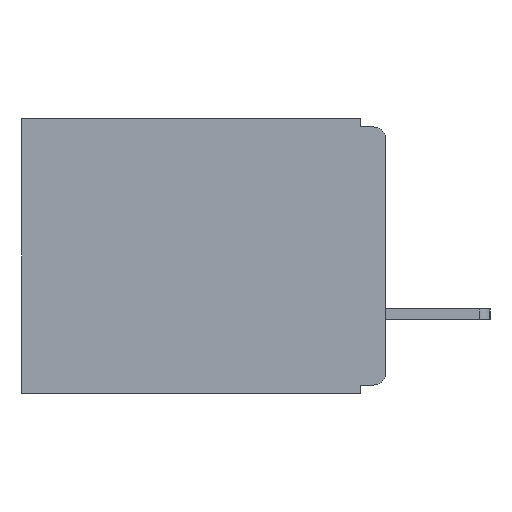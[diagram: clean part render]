
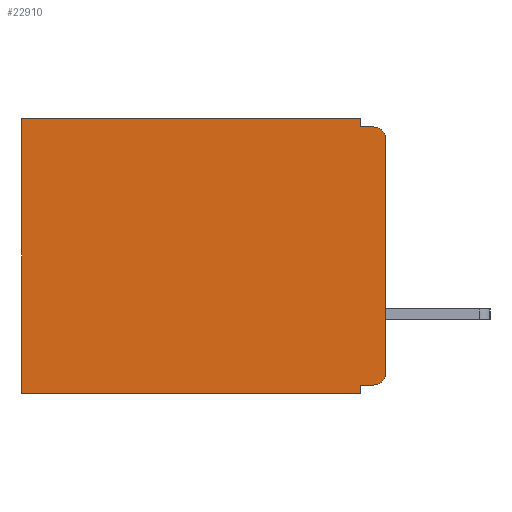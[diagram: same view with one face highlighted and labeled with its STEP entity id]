
A CAD part, left-side view. The second image highlights one B-rep face of the part: STEP entity #22910.
In plain terms, the highlighted planar face has unit normal (-1, 0, 0).
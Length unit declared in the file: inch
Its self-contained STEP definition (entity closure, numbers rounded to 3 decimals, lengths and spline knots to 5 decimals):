
#33 = EDGE_CURVE ( 'NONE', #7114, #3083, #21932, .T. ) ;
#176 = ORIENTED_EDGE ( 'NONE', *, *, #8968, .T. ) ;
#306 = LINE ( 'NONE', #16758, #4225 ) ;
#610 = CARTESIAN_POINT ( 'NONE',  ( 0.3, 0., -0.33 ) ) ;
#956 = EDGE_LOOP ( 'NONE', ( #25468, #28493, #5058, #9358, #176, #7870, #13820, #5344, #19461, #2371 ) ) ;
#1788 = VERTEX_POINT ( 'NONE', #25112 ) ;
#1789 = LINE ( 'NONE', #610, #13122 ) ;
#2048 = CARTESIAN_POINT ( 'NONE',  ( 0.3, 0.437, 0. ) ) ;
#2189 = CARTESIAN_POINT ( 'NONE',  ( 0.3, 0., -0.33 ) ) ;
#2371 = ORIENTED_EDGE ( 'NONE', *, *, #14044, .T. ) ;
#3065 = CIRCLE ( 'NONE', #7094, 0.015 ) ;
#3083 = VERTEX_POINT ( 'NONE', #17396 ) ;
#3307 = VECTOR ( 'NONE', #19195, 39.37008 ) ;
#3341 = CARTESIAN_POINT ( 'NONE',  ( 0.3, 0., -0.32 ) ) ;
#3939 = EDGE_CURVE ( 'NONE', #10313, #7800, #22770, .T. ) ;
#4132 = AXIS2_PLACEMENT_3D ( 'NONE', #9442, #25284, #11703 ) ;
#4225 = VECTOR ( 'NONE', #16646, 39.37008 ) ;
#4572 = CARTESIAN_POINT ( 'NONE',  ( 0.3, 0.031, -0.01 ) ) ;
#5058 = ORIENTED_EDGE ( 'NONE', *, *, #23156, .F. ) ;
#5195 = CARTESIAN_POINT ( 'NONE',  ( 0.3, 0., -0.305 ) ) ;
#5344 = ORIENTED_EDGE ( 'NONE', *, *, #20759, .F. ) ;
#6244 = VERTEX_POINT ( 'NONE', #16703 ) ;
#6984 = LINE ( 'NONE', #2189, #18333 ) ;
#7094 = AXIS2_PLACEMENT_3D ( 'NONE', #12845, #28700, #15104 ) ;
#7114 = VERTEX_POINT ( 'NONE', #10068 ) ;
#7800 = VERTEX_POINT ( 'NONE', #20001 ) ;
#7870 = ORIENTED_EDGE ( 'NONE', *, *, #3939, .T. ) ;
#8241 = FACE_OUTER_BOUND ( 'NONE', #956, .T. ) ;
#8554 = EDGE_CURVE ( 'NONE', #6244, #28849, #27613, .T. ) ;
#8968 = EDGE_CURVE ( 'NONE', #6244, #10313, #306, .T. ) ;
#9358 = ORIENTED_EDGE ( 'NONE', *, *, #8554, .F. ) ;
#9442 = CARTESIAN_POINT ( 'NONE',  ( 0.3, 0., -0.33 ) ) ;
#10068 = CARTESIAN_POINT ( 'NONE',  ( 0.3, 0., -0.025 ) ) ;
#10313 = VERTEX_POINT ( 'NONE', #2048 ) ;
#10722 = VECTOR ( 'NONE', #27447, 39.37008 ) ;
#11205 = VERTEX_POINT ( 'NONE', #5195 ) ;
#11414 = DIRECTION ( 'NONE',  ( 0., 0., -1. ) ) ;
#11703 = DIRECTION ( 'NONE',  ( 0., 0., -1. ) ) ;
#12845 = CARTESIAN_POINT ( 'NONE',  ( 0.3, 0.015, -0.305 ) ) ;
#13122 = VECTOR ( 'NONE', #14148, 39.37008 ) ;
#13148 = LINE ( 'NONE', #21844, #18502 ) ;
#13820 = ORIENTED_EDGE ( 'NONE', *, *, #23526, .F. ) ;
#14006 = CARTESIAN_POINT ( 'NONE',  ( 0.3, 0.031, -0.33 ) ) ;
#14044 = EDGE_CURVE ( 'NONE', #1788, #11205, #3065, .T. ) ;
#14148 = DIRECTION ( 'NONE',  ( 0., 1., 0. ) ) ;
#14203 = VERTEX_POINT ( 'NONE', #24721 ) ;
#15104 = DIRECTION ( 'NONE',  ( 0., 0., -1. ) ) ;
#16046 = EDGE_CURVE ( 'NONE', #1788, #21281, #28097, .T. ) ;
#16646 = DIRECTION ( 'NONE',  ( 0., 1., 0. ) ) ;
#16703 = CARTESIAN_POINT ( 'NONE',  ( 0.3, 0.031, 0. ) ) ;
#16758 = CARTESIAN_POINT ( 'NONE',  ( 0.3, 0., 0. ) ) ;
#17396 = CARTESIAN_POINT ( 'NONE',  ( 0.3, 0.015, -0.01 ) ) ;
#17722 = CARTESIAN_POINT ( 'NONE',  ( 0.3, 0.437, -0.33 ) ) ;
#17834 = LINE ( 'NONE', #14006, #22415 ) ;
#18333 = VECTOR ( 'NONE', #29198, 39.37008 ) ;
#18502 = VECTOR ( 'NONE', #24095, 39.37008 ) ;
#19195 = DIRECTION ( 'NONE',  ( 0., 1., 0. ) ) ;
#19461 = ORIENTED_EDGE ( 'NONE', *, *, #16046, .F. ) ;
#19625 = AXIS2_PLACEMENT_3D ( 'NONE', #28907, #20769, #11414 ) ;
#20001 = CARTESIAN_POINT ( 'NONE',  ( 0.3, 0.437, -0.33 ) ) ;
#20580 = PLANE ( 'NONE',  #4132 ) ;
#20759 = EDGE_CURVE ( 'NONE', #21281, #14203, #17834, .T. ) ;
#20769 = DIRECTION ( 'NONE',  ( -1., 0., 0. ) ) ;
#21281 = VERTEX_POINT ( 'NONE', #29148 ) ;
#21622 = VECTOR ( 'NONE', #23225, 39.37008 ) ;
#21844 = CARTESIAN_POINT ( 'NONE',  ( 0.3, 0., -0.01 ) ) ;
#21932 = CIRCLE ( 'NONE', #19625, 0.015 ) ;
#22415 = VECTOR ( 'NONE', #23057, 39.37008 ) ;
#22770 = LINE ( 'NONE', #17722, #10722 ) ;
#22910 = ADVANCED_FACE ( 'NONE', ( #8241 ), #20580, .F. ) ;
#23057 = DIRECTION ( 'NONE',  ( 0., 0., -1. ) ) ;
#23156 = EDGE_CURVE ( 'NONE', #28849, #3083, #13148, .T. ) ;
#23192 = CARTESIAN_POINT ( 'NONE',  ( 0.3, 0.031, 0. ) ) ;
#23225 = DIRECTION ( 'NONE',  ( 0., 0., -1. ) ) ;
#23526 = EDGE_CURVE ( 'NONE', #14203, #7800, #1789, .T. ) ;
#24095 = DIRECTION ( 'NONE',  ( 0., -1., 0. ) ) ;
#24721 = CARTESIAN_POINT ( 'NONE',  ( 0.3, 0.031, -0.33 ) ) ;
#25112 = CARTESIAN_POINT ( 'NONE',  ( 0.3, 0.015, -0.32 ) ) ;
#25284 = DIRECTION ( 'NONE',  ( 1., 0., 0. ) ) ;
#25468 = ORIENTED_EDGE ( 'NONE', *, *, #26465, .F. ) ;
#26465 = EDGE_CURVE ( 'NONE', #7114, #11205, #6984, .T. ) ;
#27447 = DIRECTION ( 'NONE',  ( 0., 0., -1. ) ) ;
#27613 = LINE ( 'NONE', #23192, #21622 ) ;
#28097 = LINE ( 'NONE', #3341, #3307 ) ;
#28493 = ORIENTED_EDGE ( 'NONE', *, *, #33, .T. ) ;
#28700 = DIRECTION ( 'NONE',  ( -1., 0., 0. ) ) ;
#28849 = VERTEX_POINT ( 'NONE', #4572 ) ;
#28907 = CARTESIAN_POINT ( 'NONE',  ( 0.3, 0.015, -0.025 ) ) ;
#29148 = CARTESIAN_POINT ( 'NONE',  ( 0.3, 0.031, -0.32 ) ) ;
#29198 = DIRECTION ( 'NONE',  ( 0., 0., -1. ) ) ;
